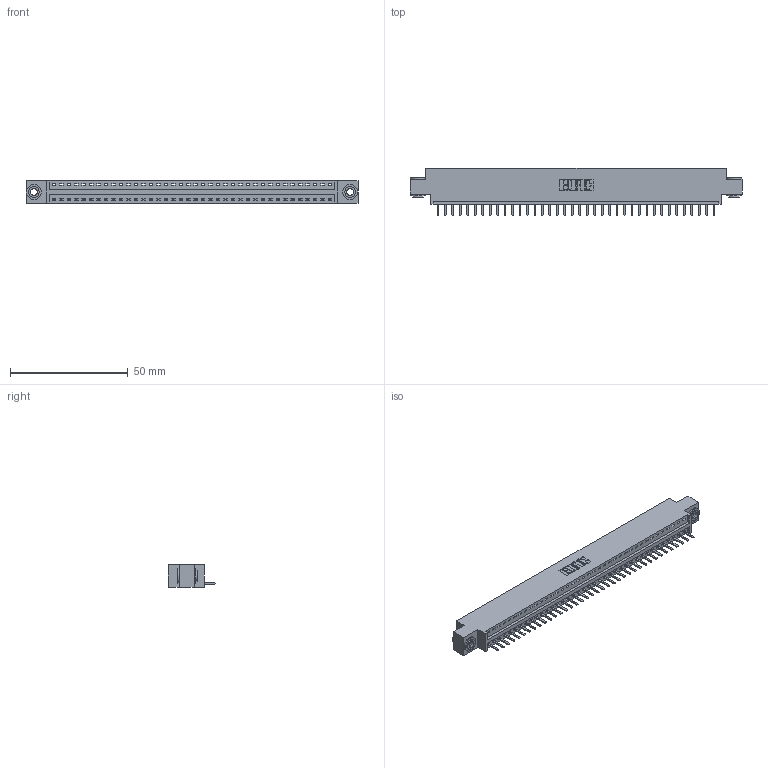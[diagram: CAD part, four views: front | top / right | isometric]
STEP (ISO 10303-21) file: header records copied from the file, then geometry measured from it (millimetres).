
FILE_DESCRIPTION (( 'STEP AP203' ), '1' );
FILE_NAME ('346-038-520-603.STEP', '2022-05-07T04:16:23', ( '' ), ( '' ), 'SwSTEP 2.0', 'SolidWorks 2020', '' );
FILE_SCHEMA (( 'CONFIG_CONTROL_DESIGN' ));
Length unit declared in the file: inch
Products named in the file (4): 346 Part_0.170 Offset - 0.156 Dia-TH; 346-038-520-603; 345-250-002_345-250-002-102; 345-292-001_345-293-120
Assembly tree (41 placements, depth 2):
  346-038-520-603
    346 Part_0.170 Offset - 0.156 Dia-TH
    345-292-001_345-293-120  x38
    345-250-002_345-250-002-102  x2
Bounding box: 141.22 x 20.02 x 9.4 mm (x, y, z)
Volume: 13228.1 mm3; surface area: 16537.1 mm2
Topology: 41 solids, 41 shells, 2534 faces, 7445 edges, 4858 vertices
Faces by surface type: plane 1700, cylinder 826, cone 8
Entity records: 25434 total; most frequent: CARTESIAN_POINT 4355, ORIENTED_EDGE 4306, DIRECTION 3863, EDGE_CURVE 2153, LINE 1841, VECTOR 1841, VERTEX_POINT 1430, AXIS2_PLACEMENT_3D 1011
